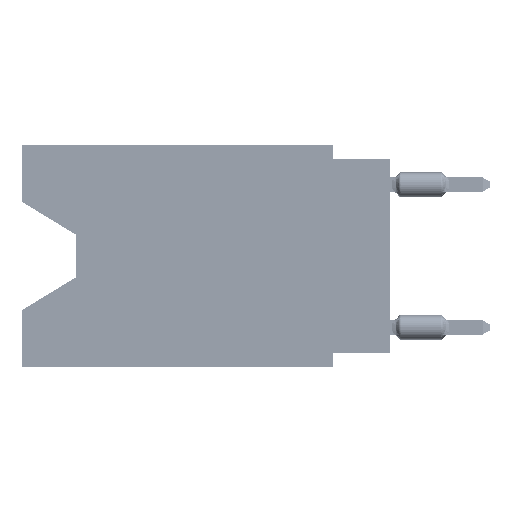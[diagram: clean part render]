
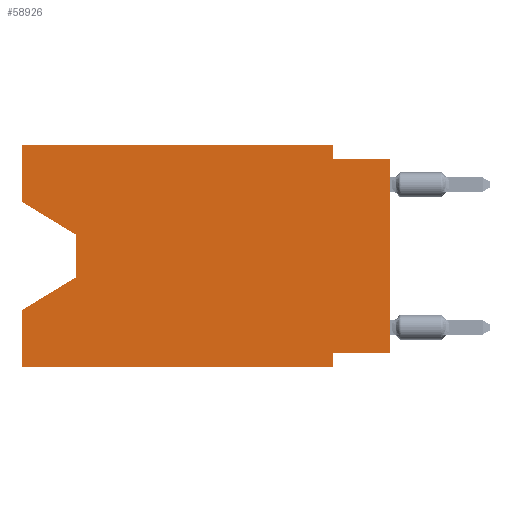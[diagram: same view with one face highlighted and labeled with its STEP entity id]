
A CAD part, left-side view. The second image highlights one B-rep face of the part: STEP entity #58926.
In plain terms, the highlighted planar face has unit normal (-1, 0, 0).
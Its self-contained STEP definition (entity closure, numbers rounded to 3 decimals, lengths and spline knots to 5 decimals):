
#592 = VERTEX_POINT ( 'NONE', #28768 ) ;
#2071 = LINE ( 'NONE', #25107, #13761 ) ;
#2322 = CARTESIAN_POINT ( 'NONE',  ( 0., 0.55, -0.158 ) ) ;
#3063 = DIRECTION ( 'NONE',  ( 0., 0., 1. ) ) ;
#4382 = VERTEX_POINT ( 'NONE', #2322 ) ;
#4756 = VERTEX_POINT ( 'NONE', #19979 ) ;
#4912 = ORIENTED_EDGE ( 'NONE', *, *, #13438, .T. ) ;
#5945 = CARTESIAN_POINT ( 'NONE',  ( 0., 0., -0.365 ) ) ;
#6220 = DIRECTION ( 'NONE',  ( 0., -1., 0. ) ) ;
#8358 = EDGE_CURVE ( 'NONE', #24911, #4756, #40122, .T. ) ;
#8636 = AXIS2_PLACEMENT_3D ( 'NONE', #10088, #14649, #56189 ) ;
#9719 = ORIENTED_EDGE ( 'NONE', *, *, #12542, .F. ) ;
#10088 = CARTESIAN_POINT ( 'NONE',  ( 0., 0.645, 0. ) ) ;
#10221 = CARTESIAN_POINT ( 'NONE',  ( 0., 0.645, -0.10025 ) ) ;
#10934 = CARTESIAN_POINT ( 'NONE',  ( 0., 0.645, 0. ) ) ;
#12095 = ORIENTED_EDGE ( 'NONE', *, *, #29699, .T. ) ;
#12124 = LINE ( 'NONE', #52564, #45979 ) ;
#12513 = CARTESIAN_POINT ( 'NONE',  ( 0., 0., -0.365 ) ) ;
#12542 = EDGE_CURVE ( 'NONE', #4756, #22455, #29659, .T. ) ;
#13438 = EDGE_CURVE ( 'NONE', #24911, #592, #25359, .T. ) ;
#13761 = VECTOR ( 'NONE', #32997, 39.37008 ) ;
#13772 = ORIENTED_EDGE ( 'NONE', *, *, #35745, .F. ) ;
#13832 = LINE ( 'NONE', #71224, #59392 ) ;
#14649 = DIRECTION ( 'NONE',  ( 1., 0., 0. ) ) ;
#15378 = CARTESIAN_POINT ( 'NONE',  ( 0., 0.645, 0. ) ) ;
#16066 = LINE ( 'NONE', #39116, #67753 ) ;
#16966 = LINE ( 'NONE', #40015, #19485 ) ;
#17819 = DIRECTION ( 'NONE',  ( 0., 1., 0. ) ) ;
#18185 = CARTESIAN_POINT ( 'NONE',  ( 0., 0.55, -0.232 ) ) ;
#19485 = VECTOR ( 'NONE', #74013, 39.37008 ) ;
#19979 = CARTESIAN_POINT ( 'NONE',  ( 0., 0.1, -0.365 ) ) ;
#20349 = VERTEX_POINT ( 'NONE', #38743 ) ;
#22150 = VERTEX_POINT ( 'NONE', #10221 ) ;
#22455 = VERTEX_POINT ( 'NONE', #37004 ) ;
#22891 = ORIENTED_EDGE ( 'NONE', *, *, #8358, .F. ) ;
#24570 = ORIENTED_EDGE ( 'NONE', *, *, #58635, .F. ) ;
#24911 = VERTEX_POINT ( 'NONE', #5945 ) ;
#25107 = CARTESIAN_POINT ( 'NONE',  ( 0., 0.55, -0.232 ) ) ;
#25359 = LINE ( 'NONE', #60464, #36418 ) ;
#28618 = DIRECTION ( 'NONE',  ( 0., -0.855, -0.519 ) ) ;
#28768 = CARTESIAN_POINT ( 'NONE',  ( 0., 0., -0.025 ) ) ;
#29659 = LINE ( 'NONE', #41004, #54372 ) ;
#29699 = EDGE_CURVE ( 'NONE', #70647, #22455, #34944, .T. ) ;
#30401 = CARTESIAN_POINT ( 'NONE',  ( 0., 0.645, -0.39 ) ) ;
#30997 = CARTESIAN_POINT ( 'NONE',  ( 0., 0.1, 0. ) ) ;
#32997 = DIRECTION ( 'NONE',  ( 0., 0.855, -0.519 ) ) ;
#33596 = EDGE_CURVE ( 'NONE', #22150, #45103, #56658, .T. ) ;
#34944 = LINE ( 'NONE', #30401, #64930 ) ;
#35745 = EDGE_CURVE ( 'NONE', #45103, #71358, #16066, .T. ) ;
#36418 = VECTOR ( 'NONE', #3063, 39.37008 ) ;
#36683 = EDGE_CURVE ( 'NONE', #20349, #592, #13832, .T. ) ;
#37004 = CARTESIAN_POINT ( 'NONE',  ( 0., 0.1, -0.39 ) ) ;
#38743 = CARTESIAN_POINT ( 'NONE',  ( 0., 0.1, -0.025 ) ) ;
#39116 = CARTESIAN_POINT ( 'NONE',  ( 0., 0.645, 0. ) ) ;
#40015 = CARTESIAN_POINT ( 'NONE',  ( 0., 0.645, 0. ) ) ;
#40122 = LINE ( 'NONE', #12513, #68433 ) ;
#41004 = CARTESIAN_POINT ( 'NONE',  ( 0., 0.1, -0.39 ) ) ;
#42837 = LINE ( 'NONE', #60548, #51374 ) ;
#43075 = ORIENTED_EDGE ( 'NONE', *, *, #51985, .T. ) ;
#43383 = FACE_OUTER_BOUND ( 'NONE', #72066, .T. ) ;
#45103 = VERTEX_POINT ( 'NONE', #15378 ) ;
#45273 = CARTESIAN_POINT ( 'NONE',  ( 0., 0.645, -0.10025 ) ) ;
#45979 = VECTOR ( 'NONE', #63127, 39.37008 ) ;
#46000 = VECTOR ( 'NONE', #49892, 39.37008 ) ;
#47846 = DIRECTION ( 'NONE',  ( 0., -1., 0. ) ) ;
#48184 = ORIENTED_EDGE ( 'NONE', *, *, #63538, .T. ) ;
#49251 = DIRECTION ( 'NONE',  ( 0., 0., -1. ) ) ;
#49892 = DIRECTION ( 'NONE',  ( 0., 0., 1. ) ) ;
#50417 = CARTESIAN_POINT ( 'NONE',  ( 0., 0.645, -0.39 ) ) ;
#51374 = VECTOR ( 'NONE', #49251, 39.37008 ) ;
#51985 = EDGE_CURVE ( 'NONE', #22150, #4382, #69750, .T. ) ;
#52564 = CARTESIAN_POINT ( 'NONE',  ( 0., 0.1, 0. ) ) ;
#53471 = CARTESIAN_POINT ( 'NONE',  ( 0., 0.645, -0.28975 ) ) ;
#54372 = VECTOR ( 'NONE', #69318, 39.37008 ) ;
#54978 = VECTOR ( 'NONE', #28618, 39.37008 ) ;
#56189 = DIRECTION ( 'NONE',  ( 0., 0., -1. ) ) ;
#56459 = VERTEX_POINT ( 'NONE', #53471 ) ;
#56658 = LINE ( 'NONE', #10934, #46000 ) ;
#58199 = EDGE_CURVE ( 'NONE', #71358, #20349, #12124, .T. ) ;
#58635 = EDGE_CURVE ( 'NONE', #70647, #56459, #16966, .T. ) ;
#58926 = ADVANCED_FACE ( 'NONE', ( #43383 ), #66386, .F. ) ;
#59392 = VECTOR ( 'NONE', #47846, 39.37008 ) ;
#60464 = CARTESIAN_POINT ( 'NONE',  ( 0., 0., 0. ) ) ;
#60548 = CARTESIAN_POINT ( 'NONE',  ( 0., 0.55, -0.158 ) ) ;
#62138 = DIRECTION ( 'NONE',  ( 0., -1., 0. ) ) ;
#63037 = ORIENTED_EDGE ( 'NONE', *, *, #73280, .T. ) ;
#63127 = DIRECTION ( 'NONE',  ( 0., 0., -1. ) ) ;
#63538 = EDGE_CURVE ( 'NONE', #4382, #63738, #42837, .T. ) ;
#63738 = VERTEX_POINT ( 'NONE', #18185 ) ;
#64930 = VECTOR ( 'NONE', #6220, 39.37008 ) ;
#65017 = ORIENTED_EDGE ( 'NONE', *, *, #36683, .F. ) ;
#65979 = ORIENTED_EDGE ( 'NONE', *, *, #58199, .F. ) ;
#66386 = PLANE ( 'NONE',  #8636 ) ;
#67753 = VECTOR ( 'NONE', #62138, 39.37008 ) ;
#68433 = VECTOR ( 'NONE', #17819, 39.37008 ) ;
#69318 = DIRECTION ( 'NONE',  ( 0., 0., -1. ) ) ;
#69750 = LINE ( 'NONE', #45273, #54978 ) ;
#69857 = ORIENTED_EDGE ( 'NONE', *, *, #33596, .F. ) ;
#70647 = VERTEX_POINT ( 'NONE', #50417 ) ;
#71224 = CARTESIAN_POINT ( 'NONE',  ( 0., 0., -0.025 ) ) ;
#71358 = VERTEX_POINT ( 'NONE', #30997 ) ;
#72066 = EDGE_LOOP ( 'NONE', ( #43075, #48184, #63037, #24570, #12095, #9719, #22891, #4912, #65017, #65979, #13772, #69857 ) ) ;
#73280 = EDGE_CURVE ( 'NONE', #63738, #56459, #2071, .T. ) ;
#74013 = DIRECTION ( 'NONE',  ( 0., 0., 1. ) ) ;
